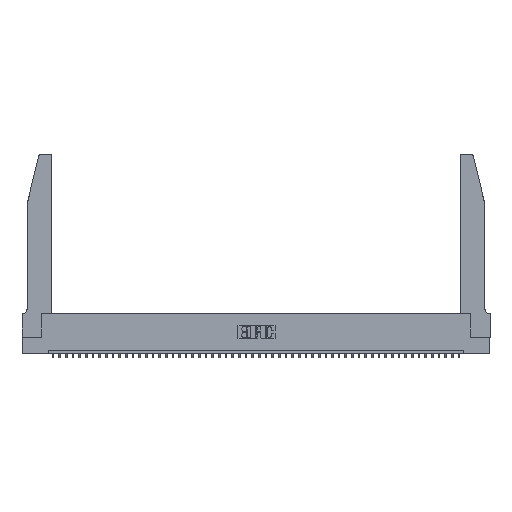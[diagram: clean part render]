
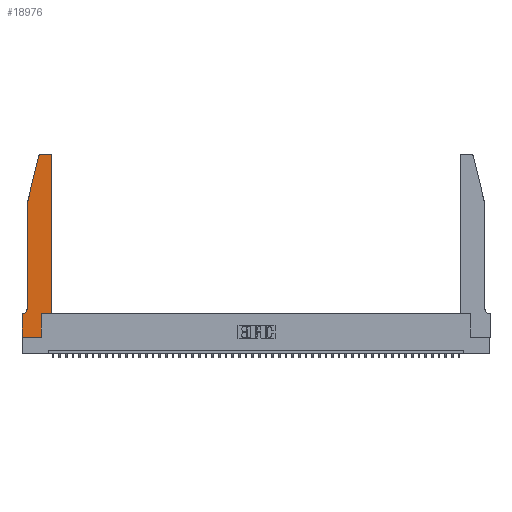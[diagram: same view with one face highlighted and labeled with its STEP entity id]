
A CAD part, top view. The second image highlights one B-rep face of the part: STEP entity #18976.
In plain terms, the highlighted planar face has unit normal (0, 0, 1).
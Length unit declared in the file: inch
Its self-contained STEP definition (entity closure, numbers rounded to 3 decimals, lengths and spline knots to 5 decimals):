
#621 = VECTOR ( 'NONE', #9437, 39.37008 ) ;
#832 = ORIENTED_EDGE ( 'NONE', *, *, #14149, .T. ) ;
#938 = EDGE_CURVE ( 'NONE', #39040, #13712, #21705, .T. ) ;
#1122 = LINE ( 'NONE', #27601, #14064 ) ;
#1272 = DIRECTION ( 'NONE',  ( 1., 0., 0. ) ) ;
#1383 = EDGE_CURVE ( 'NONE', #39645, #27485, #40042, .T. ) ;
#1455 = CARTESIAN_POINT ( 'NONE',  ( 0.2865, 0.35, 0.37 ) ) ;
#2445 = EDGE_CURVE ( 'NONE', #12627, #19482, #19109, .T. ) ;
#2761 = DIRECTION ( 'NONE',  ( 1., 0., 0. ) ) ;
#3022 = LINE ( 'NONE', #27392, #37779 ) ;
#3712 = CARTESIAN_POINT ( 'NONE',  ( 0.25487, 2.72718, 0.37 ) ) ;
#4167 = CARTESIAN_POINT ( 'NONE',  ( 0.284, 2.75, 0.37 ) ) ;
#4571 = VERTEX_POINT ( 'NONE', #3712 ) ;
#4579 = LINE ( 'NONE', #14830, #11631 ) ;
#4750 = DIRECTION ( 'NONE',  ( 1., 0., 0. ) ) ;
#4855 = EDGE_CURVE ( 'NONE', #41578, #12627, #28977, .T. ) ;
#5561 = EDGE_CURVE ( 'NONE', #17026, #4571, #33651, .T. ) ;
#5577 = DIRECTION ( 'NONE',  ( 0., 0., 1. ) ) ;
#6715 = CARTESIAN_POINT ( 'NONE',  ( 0.2865, 0.35, 0.37 ) ) ;
#6835 = CARTESIAN_POINT ( 'NONE',  ( 0., 0.35, 0.37 ) ) ;
#7290 = ORIENTED_EDGE ( 'NONE', *, *, #2445, .T. ) ;
#9437 = DIRECTION ( 'NONE',  ( -1., 0., 0. ) ) ;
#9922 = VECTOR ( 'NONE', #37056, 39.37008 ) ;
#11273 = EDGE_LOOP ( 'NONE', ( #46548, #26945, #39338, #41432, #16819, #34054, #832, #21809, #13013, #13334, #43989, #7290 ) ) ;
#11570 = CARTESIAN_POINT ( 'NONE',  ( 0.4505, 2.72, 0.37 ) ) ;
#11631 = VECTOR ( 'NONE', #39508, 39.37008 ) ;
#11777 = VERTEX_POINT ( 'NONE', #27617 ) ;
#12023 = CARTESIAN_POINT ( 'NONE',  ( 0.0055, 0.35, 0.37 ) ) ;
#12196 = EDGE_CURVE ( 'NONE', #19482, #17026, #33665, .T. ) ;
#12474 = CARTESIAN_POINT ( 'NONE',  ( 0., 0., 0.37 ) ) ;
#12627 = VERTEX_POINT ( 'NONE', #11570 ) ;
#12751 = DIRECTION ( 'NONE',  ( 1., 0., 0. ) ) ;
#13013 = ORIENTED_EDGE ( 'NONE', *, *, #1383, .T. ) ;
#13334 = ORIENTED_EDGE ( 'NONE', *, *, #32355, .T. ) ;
#13516 = DIRECTION ( 'NONE',  ( 0., -1., 0. ) ) ;
#13712 = VERTEX_POINT ( 'NONE', #6835 ) ;
#13752 = EDGE_CURVE ( 'NONE', #11777, #21237, #4579, .T. ) ;
#14064 = VECTOR ( 'NONE', #4750, 39.37008 ) ;
#14149 = EDGE_CURVE ( 'NONE', #13712, #38473, #29289, .T. ) ;
#14735 = AXIS2_PLACEMENT_3D ( 'NONE', #24088, #5577, #43359 ) ;
#14830 = CARTESIAN_POINT ( 'NONE',  ( 0.0755, 2., 0.37 ) ) ;
#15013 = CARTESIAN_POINT ( 'NONE',  ( 0.0755, 0.35, 0.37 ) ) ;
#16819 = ORIENTED_EDGE ( 'NONE', *, *, #39678, .T. ) ;
#16996 = LINE ( 'NONE', #35352, #44843 ) ;
#17026 = VERTEX_POINT ( 'NONE', #4167 ) ;
#18976 = ADVANCED_FACE ( 'NONE', ( #22234 ), #31867, .T. ) ;
#19109 = CIRCLE ( 'NONE', #23070, 0.03 ) ;
#19199 = VECTOR ( 'NONE', #13516, 39.37008 ) ;
#19482 = VERTEX_POINT ( 'NONE', #45948 ) ;
#20612 = CARTESIAN_POINT ( 'NONE',  ( 0.2605, 2.75, 0.37 ) ) ;
#20750 = AXIS2_PLACEMENT_3D ( 'NONE', #23099, #27006, #1272 ) ;
#21140 = DIRECTION ( 'NONE',  ( 0., 0., -1. ) ) ;
#21237 = VERTEX_POINT ( 'NONE', #26892 ) ;
#21294 = CARTESIAN_POINT ( 'NONE',  ( 0.0055, 0.42, 0.37 ) ) ;
#21299 = VECTOR ( 'NONE', #32595, 39.37008 ) ;
#21705 = LINE ( 'NONE', #15013, #30506 ) ;
#21809 = ORIENTED_EDGE ( 'NONE', *, *, #48012, .T. ) ;
#22234 = FACE_OUTER_BOUND ( 'NONE', #11273, .T. ) ;
#23070 = AXIS2_PLACEMENT_3D ( 'NONE', #47918, #25219, #2761 ) ;
#23099 = CARTESIAN_POINT ( 'NONE',  ( 0., 0.35, 0.37 ) ) ;
#24088 = CARTESIAN_POINT ( 'NONE',  ( 0.284, 2.72, 0.37 ) ) ;
#25219 = DIRECTION ( 'NONE',  ( 0., 0., 1. ) ) ;
#26324 = DIRECTION ( 'NONE',  ( -1., 0., 0. ) ) ;
#26892 = CARTESIAN_POINT ( 'NONE',  ( 0.0755, 0.42, 0.37 ) ) ;
#26945 = ORIENTED_EDGE ( 'NONE', *, *, #5561, .T. ) ;
#27006 = DIRECTION ( 'NONE',  ( 0., 0., 1. ) ) ;
#27392 = CARTESIAN_POINT ( 'NONE',  ( 0.4505, 0.35, 0.37 ) ) ;
#27485 = VERTEX_POINT ( 'NONE', #1455 ) ;
#27601 = CARTESIAN_POINT ( 'NONE',  ( 0., 0., 0.37 ) ) ;
#27617 = CARTESIAN_POINT ( 'NONE',  ( 0.0755, 2., 0.37 ) ) ;
#28783 = CARTESIAN_POINT ( 'NONE',  ( 0.4505, 0.35, 0.37 ) ) ;
#28977 = LINE ( 'NONE', #28783, #21299 ) ;
#29289 = LINE ( 'NONE', #12474, #19199 ) ;
#30506 = VECTOR ( 'NONE', #26324, 39.37008 ) ;
#31867 = PLANE ( 'NONE',  #20750 ) ;
#32355 = EDGE_CURVE ( 'NONE', #27485, #41578, #3022, .T. ) ;
#32595 = DIRECTION ( 'NONE',  ( 0., 1., 0. ) ) ;
#32707 = DIRECTION ( 'NONE',  ( -1., 0., 0. ) ) ;
#33651 = CIRCLE ( 'NONE', #14735, 0.03 ) ;
#33665 = LINE ( 'NONE', #20612, #621 ) ;
#34037 = AXIS2_PLACEMENT_3D ( 'NONE', #21294, #21140, #32707 ) ;
#34054 = ORIENTED_EDGE ( 'NONE', *, *, #938, .T. ) ;
#35352 = CARTESIAN_POINT ( 'NONE',  ( 0.0755, 2., 0.37 ) ) ;
#36066 = CARTESIAN_POINT ( 'NONE',  ( 0., 0., 0.37 ) ) ;
#37056 = DIRECTION ( 'NONE',  ( 0., 1., 0. ) ) ;
#37779 = VECTOR ( 'NONE', #12751, 39.37008 ) ;
#38473 = VERTEX_POINT ( 'NONE', #36066 ) ;
#39040 = VERTEX_POINT ( 'NONE', #12023 ) ;
#39066 = EDGE_CURVE ( 'NONE', #4571, #11777, #16996, .T. ) ;
#39338 = ORIENTED_EDGE ( 'NONE', *, *, #39066, .T. ) ;
#39397 = CIRCLE ( 'NONE', #34037, 0.07 ) ;
#39508 = DIRECTION ( 'NONE',  ( 0., -1., 0. ) ) ;
#39645 = VERTEX_POINT ( 'NONE', #43317 ) ;
#39678 = EDGE_CURVE ( 'NONE', #21237, #39040, #39397, .T. ) ;
#40042 = LINE ( 'NONE', #6715, #9922 ) ;
#40336 = CARTESIAN_POINT ( 'NONE',  ( 0.4505, 0.35, 0.37 ) ) ;
#41432 = ORIENTED_EDGE ( 'NONE', *, *, #13752, .T. ) ;
#41578 = VERTEX_POINT ( 'NONE', #40336 ) ;
#43317 = CARTESIAN_POINT ( 'NONE',  ( 0.2865, 0., 0.37 ) ) ;
#43359 = DIRECTION ( 'NONE',  ( 1., 0., 0. ) ) ;
#43989 = ORIENTED_EDGE ( 'NONE', *, *, #4855, .T. ) ;
#44843 = VECTOR ( 'NONE', #47090, 39.37008 ) ;
#45948 = CARTESIAN_POINT ( 'NONE',  ( 0.4205, 2.75, 0.37 ) ) ;
#46548 = ORIENTED_EDGE ( 'NONE', *, *, #12196, .T. ) ;
#47090 = DIRECTION ( 'NONE',  ( -0.239, -0.971, 0. ) ) ;
#47918 = CARTESIAN_POINT ( 'NONE',  ( 0.4205, 2.72, 0.37 ) ) ;
#48012 = EDGE_CURVE ( 'NONE', #38473, #39645, #1122, .T. ) ;
